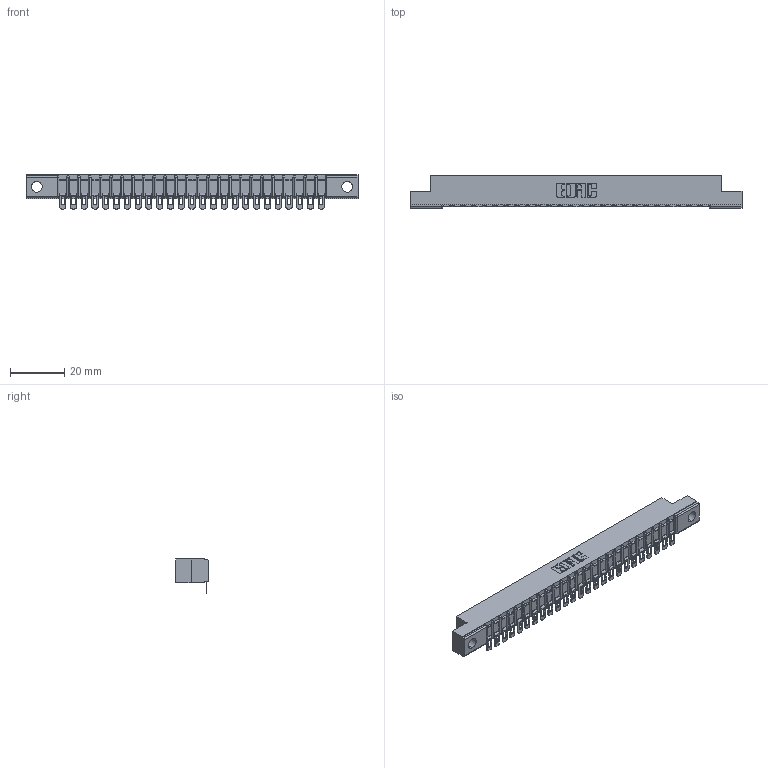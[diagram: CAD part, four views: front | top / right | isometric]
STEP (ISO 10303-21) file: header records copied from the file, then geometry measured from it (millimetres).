
FILE_DESCRIPTION (( 'STEP AP203' ), '1' );
FILE_NAME ('357-025-454-104.STEP', '2020-10-01T15:52:23', ( '' ), ( '' ), 'SwSTEP 2.0', 'SolidWorks 2020', '' );
FILE_SCHEMA (( 'CONFIG_CONTROL_DESIGN' ));
Length unit declared in the file: inch
Products named in the file (3): 357-025-454-104; 307-290-002_554; 307 Part_.156 Dia Mounting Holes
Assembly tree (26 placements, depth 2):
  357-025-454-104
    307 Part_.156 Dia Mounting Holes
    307-290-002_554  x25
Bounding box: 122.07 x 12.01 x 12.52 mm (x, y, z)
Volume: 7963.6 mm3; surface area: 14644.9 mm2
Topology: 26 solids, 26 shells, 2183 faces, 6684 edges, 4384 vertices
Faces by surface type: plane 1234, cylinder 897, sphere 52
Entity records: 24911 total; most frequent: CARTESIAN_POINT 4204, ORIENTED_EDGE 4192, DIRECTION 4090, EDGE_CURVE 2096, VECTOR 1598, LINE 1598, VERTEX_POINT 1360, AXIS2_PLACEMENT_3D 1246
